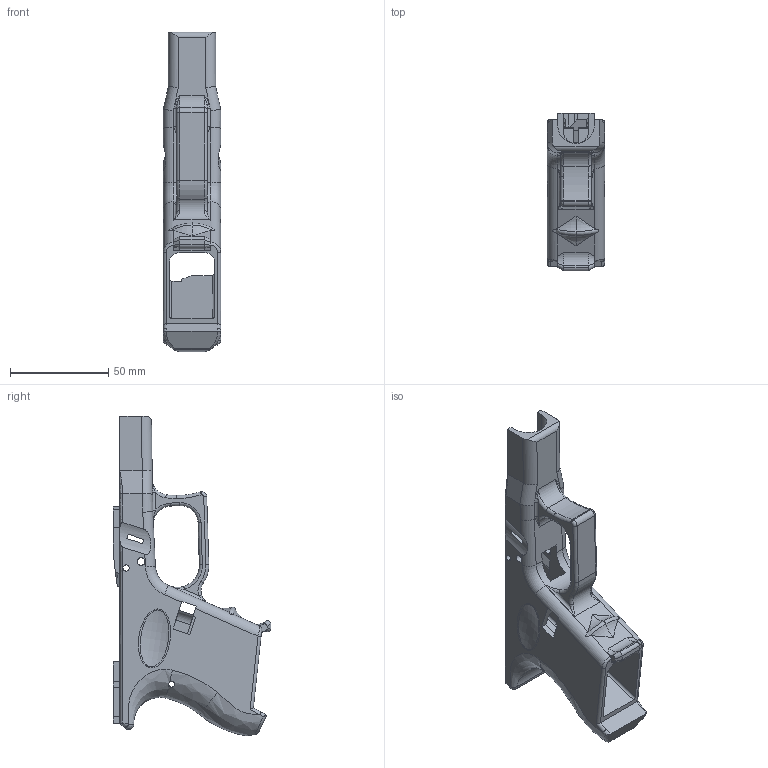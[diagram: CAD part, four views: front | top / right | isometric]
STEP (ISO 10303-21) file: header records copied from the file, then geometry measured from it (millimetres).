
FILE_DESCRIPTION (( 'STEP AP214' ), '1' );
FILE_NAME ('FRAME-RailHoles.STEP', '2018-08-01T19:03:27', ( '' ), ( '' ), 'SwSTEP 2.0', 'SolidWorks 2015', '' );
FILE_SCHEMA (( 'AUTOMOTIVE_DESIGN' ));
Length unit declared in the file: millimetre
Products named in the file (1): FRAME-RailHoles
Bounding box: 29.21 x 80.11 x 162.54 mm (x, y, z)
Volume: 81973.3 mm3; surface area: 38146.3 mm2
Topology: 1 solids, 1 shells, 320 faces, 904 edges, 565 vertices
Faces by surface type: plane 163, cylinder 81, bspline 46, torus 30
Entity records: 13226 total; most frequent: CARTESIAN_POINT 5403, ORIENTED_EDGE 1792, DIRECTION 1449, EDGE_CURVE 896, VERTEX_POINT 565, VECTOR 531, LINE 531, AXIS2_PLACEMENT_3D 459
